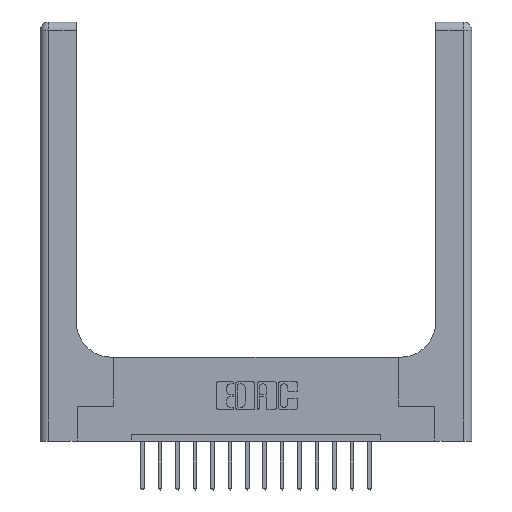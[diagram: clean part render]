
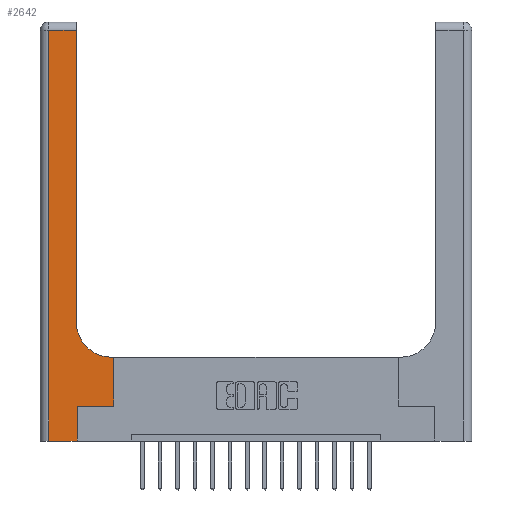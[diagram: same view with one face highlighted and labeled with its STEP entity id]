
A CAD part, top view. The second image highlights one B-rep face of the part: STEP entity #2642.
In plain terms, the highlighted planar face has unit normal (0, 0, 1).
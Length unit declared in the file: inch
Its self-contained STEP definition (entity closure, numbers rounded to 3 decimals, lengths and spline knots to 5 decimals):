
#282 = LINE ( 'NONE', #6867, #6936 ) ;
#552 = DIRECTION ( 'NONE',  ( -1., 0., 0. ) ) ;
#706 = CARTESIAN_POINT ( 'NONE',  ( 0.06, 3., 0.37 ) ) ;
#714 = EDGE_LOOP ( 'NONE', ( #8650, #12173, #4303, #1397, #13147, #11775, #16915, #17644, #5114 ) ) ;
#777 = FACE_OUTER_BOUND ( 'NONE', #714, .T. ) ;
#1397 = ORIENTED_EDGE ( 'NONE', *, *, #12621, .T. ) ;
#1803 = EDGE_CURVE ( 'NONE', #5854, #17543, #8479, .T. ) ;
#1979 = LINE ( 'NONE', #16836, #4111 ) ;
#2270 = DIRECTION ( 'NONE',  ( 1., 0., 0. ) ) ;
#2642 = ADVANCED_FACE ( 'NONE', ( #777 ), #2798, .F. ) ;
#2701 = VECTOR ( 'NONE', #552, 39.37008 ) ;
#2798 = PLANE ( 'NONE',  #17507 ) ;
#2806 = EDGE_CURVE ( 'NONE', #11010, #5854, #4628, .T. ) ;
#2936 = DIRECTION ( 'NONE',  ( 0., 1., 0. ) ) ;
#3075 = VECTOR ( 'NONE', #15941, 39.37008 ) ;
#3106 = VECTOR ( 'NONE', #17410, 39.37008 ) ;
#3494 = LINE ( 'NONE', #7788, #3075 ) ;
#3627 = CARTESIAN_POINT ( 'NONE',  ( 0.06, 0., 0.37 ) ) ;
#4008 = VERTEX_POINT ( 'NONE', #5772 ) ;
#4111 = VECTOR ( 'NONE', #6183, 39.37008 ) ;
#4303 = ORIENTED_EDGE ( 'NONE', *, *, #1803, .T. ) ;
#4458 = CARTESIAN_POINT ( 'NONE',  ( 0.528, 0.6, 0.37 ) ) ;
#4628 = LINE ( 'NONE', #15492, #2701 ) ;
#4837 = VECTOR ( 'NONE', #11683, 39.37008 ) ;
#5114 = ORIENTED_EDGE ( 'NONE', *, *, #7087, .T. ) ;
#5347 = EDGE_CURVE ( 'NONE', #8211, #8982, #16536, .T. ) ;
#5772 = CARTESIAN_POINT ( 'NONE',  ( 0.26, 0.85, 0.37 ) ) ;
#5854 = VERTEX_POINT ( 'NONE', #12147 ) ;
#6130 = CARTESIAN_POINT ( 'NONE',  ( 0.528, 0.25, 0.37 ) ) ;
#6183 = DIRECTION ( 'NONE',  ( -1., 0., 0. ) ) ;
#6514 = CARTESIAN_POINT ( 'NONE',  ( 0.265, 0.25, 0.37 ) ) ;
#6867 = CARTESIAN_POINT ( 'NONE',  ( 0.26, 3., 0.37 ) ) ;
#6936 = VECTOR ( 'NONE', #12372, 39.37008 ) ;
#7087 = EDGE_CURVE ( 'NONE', #8551, #4008, #11329, .T. ) ;
#7788 = CARTESIAN_POINT ( 'NONE',  ( 0.265, 0., 0.37 ) ) ;
#7907 = CARTESIAN_POINT ( 'NONE',  ( 0.51, 0.85, 0.37 ) ) ;
#8087 = CARTESIAN_POINT ( 'NONE',  ( 0., 3., 0.37 ) ) ;
#8154 = CARTESIAN_POINT ( 'NONE',  ( 0.265, 0., 0.37 ) ) ;
#8211 = VERTEX_POINT ( 'NONE', #15193 ) ;
#8479 = LINE ( 'NONE', #706, #4837 ) ;
#8551 = VERTEX_POINT ( 'NONE', #10292 ) ;
#8650 = ORIENTED_EDGE ( 'NONE', *, *, #13429, .T. ) ;
#8982 = VERTEX_POINT ( 'NONE', #11320 ) ;
#9075 = LINE ( 'NONE', #9386, #11255 ) ;
#9386 = CARTESIAN_POINT ( 'NONE',  ( 0., 0., 0.37 ) ) ;
#9435 = DIRECTION ( 'NONE',  ( -1., 0., 0. ) ) ;
#9516 = DIRECTION ( 'NONE',  ( 1., 0., 0. ) ) ;
#9576 = EDGE_CURVE ( 'NONE', #13966, #8551, #1979, .T. ) ;
#10292 = CARTESIAN_POINT ( 'NONE',  ( 0.51, 0.6, 0.37 ) ) ;
#10487 = DIRECTION ( 'NONE',  ( 0., 0., -1. ) ) ;
#10666 = AXIS2_PLACEMENT_3D ( 'NONE', #7907, #10487, #2270 ) ;
#10832 = DIRECTION ( 'NONE',  ( 0., 0., -1. ) ) ;
#11010 = VERTEX_POINT ( 'NONE', #11262 ) ;
#11255 = VECTOR ( 'NONE', #9516, 39.37008 ) ;
#11262 = CARTESIAN_POINT ( 'NONE',  ( 0.26, 2.94, 0.37 ) ) ;
#11320 = CARTESIAN_POINT ( 'NONE',  ( 0.528, 0.25, 0.37 ) ) ;
#11329 = CIRCLE ( 'NONE', #10666, 0.25 ) ;
#11683 = DIRECTION ( 'NONE',  ( 0., -1., 0. ) ) ;
#11775 = ORIENTED_EDGE ( 'NONE', *, *, #5347, .T. ) ;
#12147 = CARTESIAN_POINT ( 'NONE',  ( 0.06, 2.94, 0.37 ) ) ;
#12173 = ORIENTED_EDGE ( 'NONE', *, *, #2806, .T. ) ;
#12372 = DIRECTION ( 'NONE',  ( 0., 1., 0. ) ) ;
#12621 = EDGE_CURVE ( 'NONE', #17543, #13439, #9075, .T. ) ;
#13147 = ORIENTED_EDGE ( 'NONE', *, *, #14046, .T. ) ;
#13429 = EDGE_CURVE ( 'NONE', #4008, #11010, #282, .T. ) ;
#13439 = VERTEX_POINT ( 'NONE', #8154 ) ;
#13966 = VERTEX_POINT ( 'NONE', #4458 ) ;
#14046 = EDGE_CURVE ( 'NONE', #13439, #8211, #3494, .T. ) ;
#14113 = LINE ( 'NONE', #6130, #16228 ) ;
#15193 = CARTESIAN_POINT ( 'NONE',  ( 0.265, 0.25, 0.37 ) ) ;
#15492 = CARTESIAN_POINT ( 'NONE',  ( 0., 2.94, 0.37 ) ) ;
#15778 = EDGE_CURVE ( 'NONE', #8982, #13966, #14113, .T. ) ;
#15941 = DIRECTION ( 'NONE',  ( 0., 1., 0. ) ) ;
#16228 = VECTOR ( 'NONE', #2936, 39.37008 ) ;
#16536 = LINE ( 'NONE', #6514, #3106 ) ;
#16836 = CARTESIAN_POINT ( 'NONE',  ( 0.26, 0.6, 0.37 ) ) ;
#16915 = ORIENTED_EDGE ( 'NONE', *, *, #15778, .T. ) ;
#17410 = DIRECTION ( 'NONE',  ( 1., 0., 0. ) ) ;
#17507 = AXIS2_PLACEMENT_3D ( 'NONE', #8087, #10832, #9435 ) ;
#17543 = VERTEX_POINT ( 'NONE', #3627 ) ;
#17644 = ORIENTED_EDGE ( 'NONE', *, *, #9576, .T. ) ;
